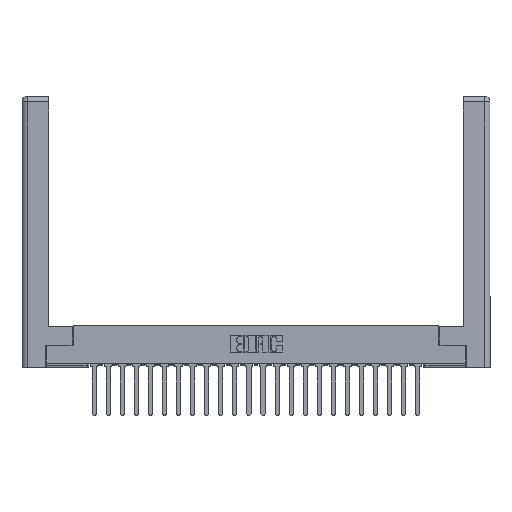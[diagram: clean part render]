
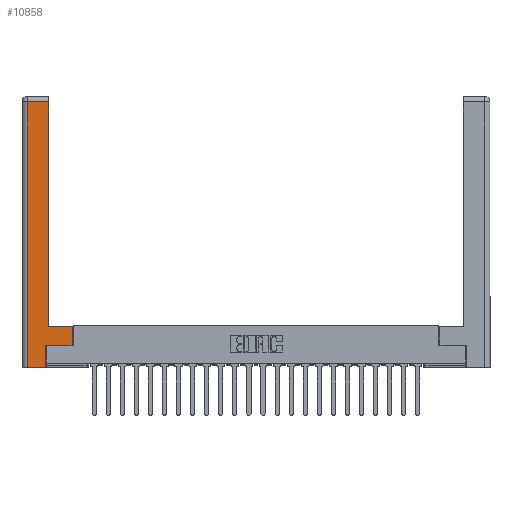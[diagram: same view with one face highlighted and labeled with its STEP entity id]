
A CAD part, top view. The second image highlights one B-rep face of the part: STEP entity #10858.
In plain terms, the highlighted planar face has unit normal (0, 0, 1).
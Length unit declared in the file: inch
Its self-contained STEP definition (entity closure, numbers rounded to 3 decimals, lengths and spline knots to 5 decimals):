
#220 = VERTEX_POINT ( 'NONE', #19173 ) ;
#475 = VERTEX_POINT ( 'NONE', #15695 ) ;
#1573 = VERTEX_POINT ( 'NONE', #20730 ) ;
#2135 = PLANE ( 'NONE',  #24424 ) ;
#2169 = ORIENTED_EDGE ( 'NONE', *, *, #3380, .T. ) ;
#2866 = EDGE_CURVE ( 'NONE', #13299, #14216, #18577, .T. ) ;
#3380 = EDGE_CURVE ( 'NONE', #1573, #21704, #15706, .T. ) ;
#4088 = EDGE_LOOP ( 'NONE', ( #2169, #15037, #19035, #18538, #8793, #14057, #20820, #18608 ) ) ;
#4257 = VECTOR ( 'NONE', #12468, 39.37008 ) ;
#4857 = DIRECTION ( 'NONE',  ( 0., -1., 0. ) ) ;
#5084 = CARTESIAN_POINT ( 'NONE',  ( 0.565, 0.245, 0. ) ) ;
#5215 = EDGE_CURVE ( 'NONE', #23372, #220, #13982, .T. ) ;
#6632 = CARTESIAN_POINT ( 'NONE',  ( 0.265, 0.245, 0. ) ) ;
#6780 = CARTESIAN_POINT ( 'NONE',  ( 0.265, 0., 0. ) ) ;
#6998 = CARTESIAN_POINT ( 'NONE',  ( 0.295, 0.45, 0. ) ) ;
#8583 = CARTESIAN_POINT ( 'NONE',  ( 0.0615, 2.94, 0. ) ) ;
#8793 = ORIENTED_EDGE ( 'NONE', *, *, #23503, .T. ) ;
#10332 = VECTOR ( 'NONE', #17410, 39.37008 ) ;
#10765 = DIRECTION ( 'NONE',  ( 0., 1., 0. ) ) ;
#10858 = ADVANCED_FACE ( 'NONE', ( #11373 ), #2135, .F. ) ;
#10953 = DIRECTION ( 'NONE',  ( 1., 0., 0. ) ) ;
#11288 = VECTOR ( 'NONE', #4857, 39.37008 ) ;
#11373 = FACE_OUTER_BOUND ( 'NONE', #4088, .T. ) ;
#11771 = VECTOR ( 'NONE', #26032, 39.37008 ) ;
#12468 = DIRECTION ( 'NONE',  ( -1., 0., 0. ) ) ;
#13084 = LINE ( 'NONE', #6998, #23233 ) ;
#13299 = VERTEX_POINT ( 'NONE', #23589 ) ;
#13969 = VECTOR ( 'NONE', #10765, 39.37008 ) ;
#13982 = LINE ( 'NONE', #5084, #23789 ) ;
#14039 = LINE ( 'NONE', #8583, #4257 ) ;
#14057 = ORIENTED_EDGE ( 'NONE', *, *, #5215, .T. ) ;
#14216 = VERTEX_POINT ( 'NONE', #25892 ) ;
#14857 = EDGE_CURVE ( 'NONE', #14216, #19392, #25746, .T. ) ;
#15037 = ORIENTED_EDGE ( 'NONE', *, *, #17501, .T. ) ;
#15366 = CARTESIAN_POINT ( 'NONE',  ( 0.295, 2.94, 0. ) ) ;
#15695 = CARTESIAN_POINT ( 'NONE',  ( 0.565, 0.45, 0. ) ) ;
#15706 = LINE ( 'NONE', #23493, #10332 ) ;
#15777 = VECTOR ( 'NONE', #22827, 39.37008 ) ;
#15838 = EDGE_CURVE ( 'NONE', #220, #475, #25067, .T. ) ;
#16297 = DIRECTION ( 'NONE',  ( -1., 0., 0. ) ) ;
#16721 = LINE ( 'NONE', #6632, #15777 ) ;
#17410 = DIRECTION ( 'NONE',  ( 0., 1., 0. ) ) ;
#17501 = EDGE_CURVE ( 'NONE', #21704, #13299, #14039, .T. ) ;
#18538 = ORIENTED_EDGE ( 'NONE', *, *, #14857, .T. ) ;
#18577 = LINE ( 'NONE', #19047, #11288 ) ;
#18608 = ORIENTED_EDGE ( 'NONE', *, *, #21530, .T. ) ;
#19035 = ORIENTED_EDGE ( 'NONE', *, *, #2866, .T. ) ;
#19047 = CARTESIAN_POINT ( 'NONE',  ( 0.0615, 0., 0. ) ) ;
#19173 = CARTESIAN_POINT ( 'NONE',  ( 0.565, 0.245, 0. ) ) ;
#19392 = VERTEX_POINT ( 'NONE', #6780 ) ;
#20183 = CARTESIAN_POINT ( 'NONE',  ( 0., 0., 0. ) ) ;
#20277 = DIRECTION ( 'NONE',  ( 0., 0., -1. ) ) ;
#20730 = CARTESIAN_POINT ( 'NONE',  ( 0.295, 0.45, 0. ) ) ;
#20820 = ORIENTED_EDGE ( 'NONE', *, *, #15838, .T. ) ;
#21530 = EDGE_CURVE ( 'NONE', #475, #1573, #13084, .T. ) ;
#21704 = VERTEX_POINT ( 'NONE', #15366 ) ;
#22127 = CARTESIAN_POINT ( 'NONE',  ( 0.265, 0., 0. ) ) ;
#22386 = CARTESIAN_POINT ( 'NONE',  ( 0.265, 0.245, 0. ) ) ;
#22827 = DIRECTION ( 'NONE',  ( 0., 1., 0. ) ) ;
#23190 = CARTESIAN_POINT ( 'NONE',  ( 0.565, 0.45, 0. ) ) ;
#23233 = VECTOR ( 'NONE', #24875, 39.37008 ) ;
#23372 = VERTEX_POINT ( 'NONE', #22386 ) ;
#23493 = CARTESIAN_POINT ( 'NONE',  ( 0.295, 3., 0. ) ) ;
#23503 = EDGE_CURVE ( 'NONE', #19392, #23372, #16721, .T. ) ;
#23589 = CARTESIAN_POINT ( 'NONE',  ( 0.0615, 2.94, 0. ) ) ;
#23789 = VECTOR ( 'NONE', #10953, 39.37008 ) ;
#24424 = AXIS2_PLACEMENT_3D ( 'NONE', #20183, #20277, #16297 ) ;
#24875 = DIRECTION ( 'NONE',  ( -1., 0., 0. ) ) ;
#25067 = LINE ( 'NONE', #23190, #13969 ) ;
#25746 = LINE ( 'NONE', #22127, #11771 ) ;
#25892 = CARTESIAN_POINT ( 'NONE',  ( 0.0615, 0., 0. ) ) ;
#26032 = DIRECTION ( 'NONE',  ( 1., 0., 0. ) ) ;
